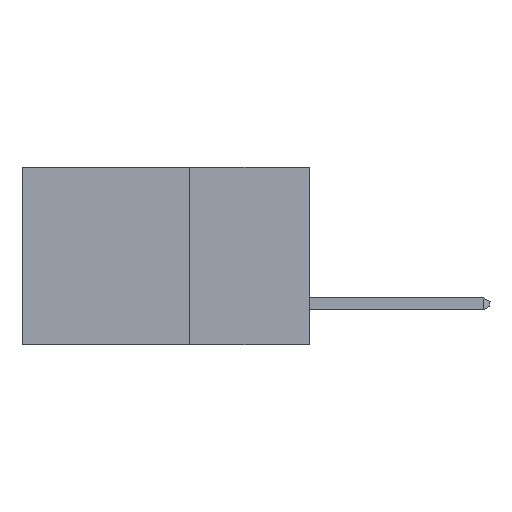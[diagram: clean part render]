
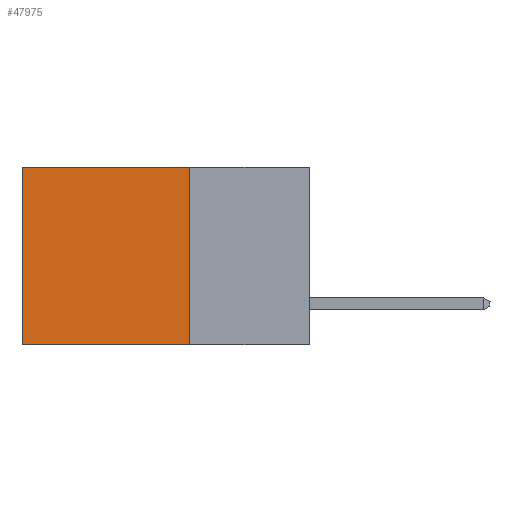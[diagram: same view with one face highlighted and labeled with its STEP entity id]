
A CAD part, left-side view. The second image highlights one B-rep face of the part: STEP entity #47975.
In plain terms, the highlighted planar face has unit normal (-1, 0, 0).
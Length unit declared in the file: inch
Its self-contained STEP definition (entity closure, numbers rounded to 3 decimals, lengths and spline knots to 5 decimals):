
#1021 = EDGE_CURVE ( 'NONE', #44928, #5477, #29417, .T. ) ;
#5477 = VERTEX_POINT ( 'NONE', #19052 ) ;
#5510 = DIRECTION ( 'NONE',  ( 0., 0., -1. ) ) ;
#6340 = VECTOR ( 'NONE', #37521, 39.37008 ) ;
#6463 = DIRECTION ( 'NONE',  ( 0., 1., 0. ) ) ;
#10552 = CARTESIAN_POINT ( 'NONE',  ( 0.2875, 0.6, 0. ) ) ;
#12261 = CARTESIAN_POINT ( 'NONE',  ( 0.2875, 0.25, 0. ) ) ;
#16306 = DIRECTION ( 'NONE',  ( 0., 1., 0. ) ) ;
#16994 = FACE_OUTER_BOUND ( 'NONE', #41594, .T. ) ;
#19051 = CARTESIAN_POINT ( 'NONE',  ( 0.2875, 0.25, -0.37 ) ) ;
#19052 = CARTESIAN_POINT ( 'NONE',  ( 0.2875, 0.6, -0.37 ) ) ;
#19800 = EDGE_CURVE ( 'NONE', #39654, #44928, #25490, .T. ) ;
#20034 = LINE ( 'NONE', #35265, #39962 ) ;
#21521 = VECTOR ( 'NONE', #29488, 39.37008 ) ;
#23617 = CARTESIAN_POINT ( 'NONE',  ( 0.2875, 0.6, 0. ) ) ;
#25490 = LINE ( 'NONE', #44725, #21521 ) ;
#26442 = ORIENTED_EDGE ( 'NONE', *, *, #19800, .F. ) ;
#28050 = ORIENTED_EDGE ( 'NONE', *, *, #43540, .T. ) ;
#28407 = VECTOR ( 'NONE', #6463, 39.37008 ) ;
#29417 = LINE ( 'NONE', #40909, #28407 ) ;
#29488 = DIRECTION ( 'NONE',  ( 0., 0., -1. ) ) ;
#29893 = ORIENTED_EDGE ( 'NONE', *, *, #45059, .T. ) ;
#31480 = DIRECTION ( 'NONE',  ( 1., 0., 0. ) ) ;
#32188 = CARTESIAN_POINT ( 'NONE',  ( 0.2875, 0.25, 0. ) ) ;
#33814 = VERTEX_POINT ( 'NONE', #23617 ) ;
#34594 = AXIS2_PLACEMENT_3D ( 'NONE', #12261, #31480, #5510 ) ;
#35265 = CARTESIAN_POINT ( 'NONE',  ( 0.2875, 0.25, 0. ) ) ;
#36647 = ORIENTED_EDGE ( 'NONE', *, *, #1021, .F. ) ;
#37521 = DIRECTION ( 'NONE',  ( 0., 0., -1. ) ) ;
#39654 = VERTEX_POINT ( 'NONE', #32188 ) ;
#39962 = VECTOR ( 'NONE', #16306, 39.37008 ) ;
#40909 = CARTESIAN_POINT ( 'NONE',  ( 0.2875, 0.25, -0.37 ) ) ;
#41594 = EDGE_LOOP ( 'NONE', ( #28050, #36647, #26442, #29893 ) ) ;
#43540 = EDGE_CURVE ( 'NONE', #33814, #5477, #44772, .T. ) ;
#44725 = CARTESIAN_POINT ( 'NONE',  ( 0.2875, 0.25, 0. ) ) ;
#44772 = LINE ( 'NONE', #10552, #6340 ) ;
#44928 = VERTEX_POINT ( 'NONE', #19051 ) ;
#45059 = EDGE_CURVE ( 'NONE', #39654, #33814, #20034, .T. ) ;
#46957 = PLANE ( 'NONE',  #34594 ) ;
#47975 = ADVANCED_FACE ( 'NONE', ( #16994 ), #46957, .F. ) ;
